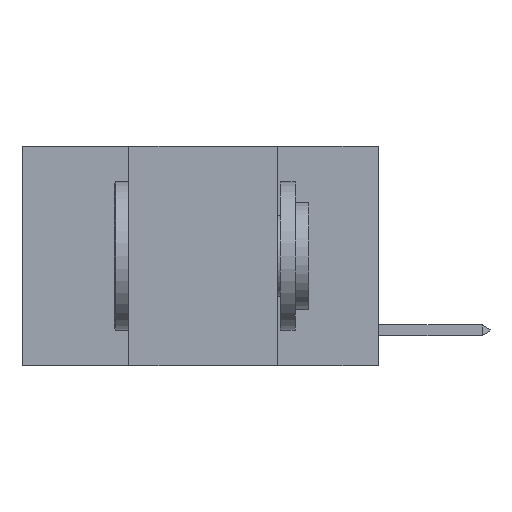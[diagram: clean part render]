
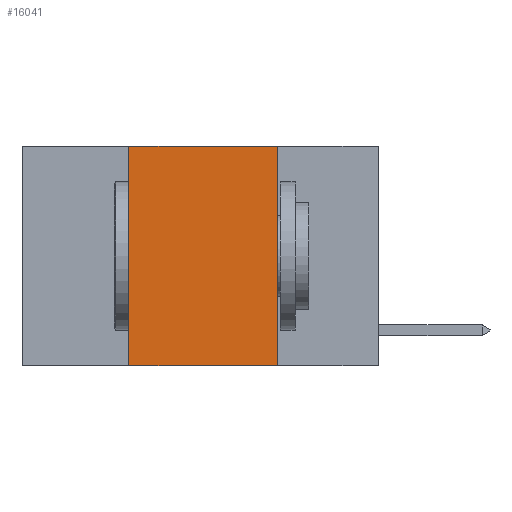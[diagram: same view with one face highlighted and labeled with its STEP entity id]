
A CAD part, left-side view. The second image highlights one B-rep face of the part: STEP entity #16041.
In plain terms, the highlighted planar face has unit normal (-1, 0, 0).
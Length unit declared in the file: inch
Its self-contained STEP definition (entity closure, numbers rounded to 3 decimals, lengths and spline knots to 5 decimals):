
#1078 = EDGE_LOOP ( 'NONE', ( #25663, #22158, #7847, #13288 ) ) ;
#3594 = LINE ( 'NONE', #9999, #18435 ) ;
#3846 = EDGE_CURVE ( 'NONE', #22294, #19851, #9731, .T. ) ;
#4038 = CARTESIAN_POINT ( 'NONE',  ( 0., 0.6, 0. ) ) ;
#4690 = LINE ( 'NONE', #14067, #9423 ) ;
#5524 = DIRECTION ( 'NONE',  ( 0., 0., 1. ) ) ;
#6197 = LINE ( 'NONE', #20015, #16158 ) ;
#7847 = ORIENTED_EDGE ( 'NONE', *, *, #22974, .F. ) ;
#8495 = EDGE_CURVE ( 'NONE', #19851, #17666, #4690, .T. ) ;
#9423 = VECTOR ( 'NONE', #22687, 39.37008 ) ;
#9440 = VECTOR ( 'NONE', #14774, 39.37008 ) ;
#9731 = LINE ( 'NONE', #18791, #9440 ) ;
#9999 = CARTESIAN_POINT ( 'NONE',  ( 0., 0.42, 0. ) ) ;
#11197 = EDGE_CURVE ( 'NONE', #23329, #17666, #6197, .T. ) ;
#12820 = FACE_OUTER_BOUND ( 'NONE', #1078, .T. ) ;
#12976 = PLANE ( 'NONE',  #20138 ) ;
#13118 = DIRECTION ( 'NONE',  ( 1., 0., 0. ) ) ;
#13288 = ORIENTED_EDGE ( 'NONE', *, *, #11197, .T. ) ;
#13482 = CARTESIAN_POINT ( 'NONE',  ( 0., 0.42, 0. ) ) ;
#14067 = CARTESIAN_POINT ( 'NONE',  ( 0., 0.17, 0. ) ) ;
#14123 = CARTESIAN_POINT ( 'NONE',  ( 0., 0.17, 0. ) ) ;
#14774 = DIRECTION ( 'NONE',  ( 0., -1., 0. ) ) ;
#16041 = ADVANCED_FACE ( 'NONE', ( #12820 ), #12976, .F. ) ;
#16158 = VECTOR ( 'NONE', #17790, 39.37008 ) ;
#17666 = VERTEX_POINT ( 'NONE', #27047 ) ;
#17790 = DIRECTION ( 'NONE',  ( 0., -1., 0. ) ) ;
#18435 = VECTOR ( 'NONE', #5524, 39.37008 ) ;
#18791 = CARTESIAN_POINT ( 'NONE',  ( 0., 0.6, 0. ) ) ;
#19851 = VERTEX_POINT ( 'NONE', #14123 ) ;
#20015 = CARTESIAN_POINT ( 'NONE',  ( 0., 0.6, -0.37 ) ) ;
#20138 = AXIS2_PLACEMENT_3D ( 'NONE', #4038, #13118, #22179 ) ;
#22158 = ORIENTED_EDGE ( 'NONE', *, *, #3846, .F. ) ;
#22179 = DIRECTION ( 'NONE',  ( 0., 0., -1. ) ) ;
#22294 = VERTEX_POINT ( 'NONE', #13482 ) ;
#22687 = DIRECTION ( 'NONE',  ( 0., 0., -1. ) ) ;
#22974 = EDGE_CURVE ( 'NONE', #23329, #22294, #3594, .T. ) ;
#23212 = CARTESIAN_POINT ( 'NONE',  ( 0., 0.42, -0.37 ) ) ;
#23329 = VERTEX_POINT ( 'NONE', #23212 ) ;
#25663 = ORIENTED_EDGE ( 'NONE', *, *, #8495, .F. ) ;
#27047 = CARTESIAN_POINT ( 'NONE',  ( 0., 0.17, -0.37 ) ) ;
